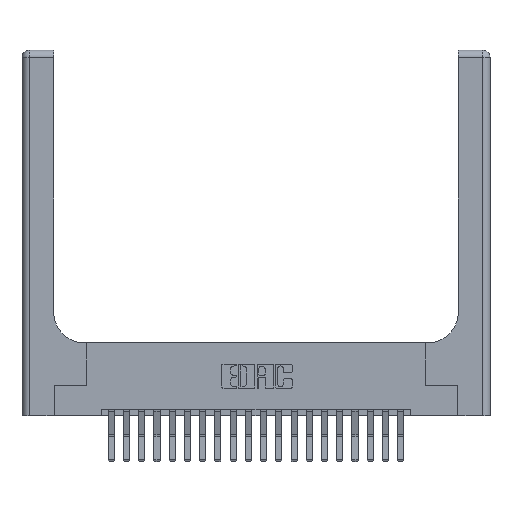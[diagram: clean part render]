
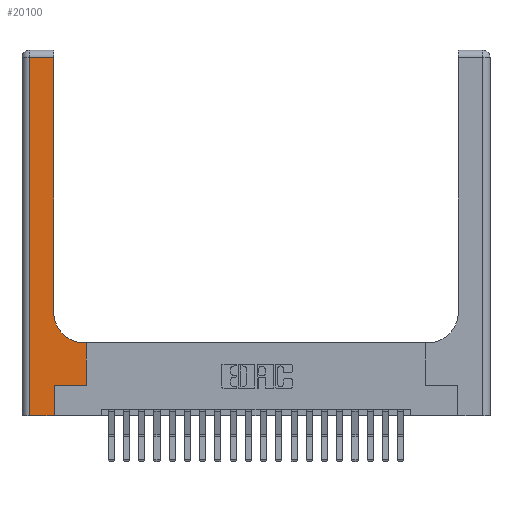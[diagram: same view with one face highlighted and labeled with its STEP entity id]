
A CAD part, top view. The second image highlights one B-rep face of the part: STEP entity #20100.
In plain terms, the highlighted planar face has unit normal (0, 0, 1).
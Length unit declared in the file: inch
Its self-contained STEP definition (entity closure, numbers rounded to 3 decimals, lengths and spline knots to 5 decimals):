
#234 = VECTOR ( 'NONE', #13671, 39.37008 ) ;
#561 = CARTESIAN_POINT ( 'NONE',  ( 0.26, 0.6, 0.37 ) ) ;
#590 = CIRCLE ( 'NONE', #10752, 0.25 ) ;
#679 = VECTOR ( 'NONE', #9015, 39.37008 ) ;
#888 = LINE ( 'NONE', #561, #679 ) ;
#981 = VECTOR ( 'NONE', #6049, 39.37008 ) ;
#1722 = CARTESIAN_POINT ( 'NONE',  ( 0.265, 0., 0.37 ) ) ;
#1819 = VERTEX_POINT ( 'NONE', #3884 ) ;
#2094 = FACE_OUTER_BOUND ( 'NONE', #9244, .T. ) ;
#2648 = CARTESIAN_POINT ( 'NONE',  ( 0., 0., 0.37 ) ) ;
#3008 = DIRECTION ( 'NONE',  ( 1., 0., 0. ) ) ;
#3083 = VERTEX_POINT ( 'NONE', #11999 ) ;
#3443 = VERTEX_POINT ( 'NONE', #10113 ) ;
#3742 = EDGE_CURVE ( 'NONE', #6792, #18751, #6155, .T. ) ;
#3884 = CARTESIAN_POINT ( 'NONE',  ( 0.528, 0.25, 0.37 ) ) ;
#4431 = EDGE_CURVE ( 'NONE', #14919, #6886, #15430, .T. ) ;
#4685 = AXIS2_PLACEMENT_3D ( 'NONE', #8678, #15389, #20233 ) ;
#4989 = EDGE_CURVE ( 'NONE', #3443, #14919, #16165, .T. ) ;
#5001 = ORIENTED_EDGE ( 'NONE', *, *, #4431, .T. ) ;
#5224 = DIRECTION ( 'NONE',  ( 0., 1., 0. ) ) ;
#5262 = ORIENTED_EDGE ( 'NONE', *, *, #3742, .T. ) ;
#5453 = DIRECTION ( 'NONE',  ( 0., 1., 0. ) ) ;
#5541 = EDGE_CURVE ( 'NONE', #6886, #6792, #6564, .T. ) ;
#5683 = EDGE_CURVE ( 'NONE', #1819, #17136, #11819, .T. ) ;
#5905 = ORIENTED_EDGE ( 'NONE', *, *, #11962, .T. ) ;
#6049 = DIRECTION ( 'NONE',  ( 0., 1., 0. ) ) ;
#6155 = LINE ( 'NONE', #2648, #15317 ) ;
#6564 = LINE ( 'NONE', #13371, #17859 ) ;
#6792 = VERTEX_POINT ( 'NONE', #8618 ) ;
#6886 = VERTEX_POINT ( 'NONE', #19608 ) ;
#7027 = EDGE_CURVE ( 'NONE', #3083, #3443, #590, .T. ) ;
#7193 = ORIENTED_EDGE ( 'NONE', *, *, #15438, .T. ) ;
#8172 = CARTESIAN_POINT ( 'NONE',  ( 0.26, 2.94, 0.37 ) ) ;
#8618 = CARTESIAN_POINT ( 'NONE',  ( 0.06, 0., 0.37 ) ) ;
#8678 = CARTESIAN_POINT ( 'NONE',  ( 0., 3., 0.37 ) ) ;
#9015 = DIRECTION ( 'NONE',  ( -1., 0., 0. ) ) ;
#9226 = CARTESIAN_POINT ( 'NONE',  ( 0.26, 3., 0.37 ) ) ;
#9244 = EDGE_LOOP ( 'NONE', ( #19111, #5001, #17368, #5262, #14146, #7193, #20048, #5905, #17726 ) ) ;
#9334 = DIRECTION ( 'NONE',  ( 1., 0., 0. ) ) ;
#10013 = CARTESIAN_POINT ( 'NONE',  ( 0.265, 0.25, 0.37 ) ) ;
#10113 = CARTESIAN_POINT ( 'NONE',  ( 0.26, 0.85, 0.37 ) ) ;
#10190 = VECTOR ( 'NONE', #5224, 39.37008 ) ;
#10411 = CARTESIAN_POINT ( 'NONE',  ( 0.265, 0.25, 0.37 ) ) ;
#10509 = LINE ( 'NONE', #10411, #15478 ) ;
#10752 = AXIS2_PLACEMENT_3D ( 'NONE', #13218, #13107, #3008 ) ;
#11695 = VERTEX_POINT ( 'NONE', #10013 ) ;
#11819 = LINE ( 'NONE', #15132, #21029 ) ;
#11962 = EDGE_CURVE ( 'NONE', #17136, #3083, #888, .T. ) ;
#11999 = CARTESIAN_POINT ( 'NONE',  ( 0.51, 0.6, 0.37 ) ) ;
#13107 = DIRECTION ( 'NONE',  ( 0., 0., -1. ) ) ;
#13218 = CARTESIAN_POINT ( 'NONE',  ( 0.51, 0.85, 0.37 ) ) ;
#13265 = DIRECTION ( 'NONE',  ( 0., -1., 0. ) ) ;
#13371 = CARTESIAN_POINT ( 'NONE',  ( 0.06, 3., 0.37 ) ) ;
#13671 = DIRECTION ( 'NONE',  ( -1., 0., 0. ) ) ;
#14146 = ORIENTED_EDGE ( 'NONE', *, *, #15577, .T. ) ;
#14919 = VERTEX_POINT ( 'NONE', #8172 ) ;
#15132 = CARTESIAN_POINT ( 'NONE',  ( 0.528, 0.25, 0.37 ) ) ;
#15317 = VECTOR ( 'NONE', #9334, 39.37008 ) ;
#15389 = DIRECTION ( 'NONE',  ( 0., 0., -1. ) ) ;
#15430 = LINE ( 'NONE', #17202, #234 ) ;
#15438 = EDGE_CURVE ( 'NONE', #11695, #1819, #10509, .T. ) ;
#15478 = VECTOR ( 'NONE', #18988, 39.37008 ) ;
#15577 = EDGE_CURVE ( 'NONE', #18751, #11695, #16671, .T. ) ;
#16165 = LINE ( 'NONE', #9226, #981 ) ;
#16671 = LINE ( 'NONE', #1722, #10190 ) ;
#16826 = PLANE ( 'NONE',  #4685 ) ;
#17117 = CARTESIAN_POINT ( 'NONE',  ( 0.528, 0.6, 0.37 ) ) ;
#17136 = VERTEX_POINT ( 'NONE', #17117 ) ;
#17202 = CARTESIAN_POINT ( 'NONE',  ( 0., 2.94, 0.37 ) ) ;
#17368 = ORIENTED_EDGE ( 'NONE', *, *, #5541, .T. ) ;
#17726 = ORIENTED_EDGE ( 'NONE', *, *, #7027, .T. ) ;
#17859 = VECTOR ( 'NONE', #13265, 39.37008 ) ;
#18446 = CARTESIAN_POINT ( 'NONE',  ( 0.265, 0., 0.37 ) ) ;
#18751 = VERTEX_POINT ( 'NONE', #18446 ) ;
#18988 = DIRECTION ( 'NONE',  ( 1., 0., 0. ) ) ;
#19111 = ORIENTED_EDGE ( 'NONE', *, *, #4989, .T. ) ;
#19608 = CARTESIAN_POINT ( 'NONE',  ( 0.06, 2.94, 0.37 ) ) ;
#20048 = ORIENTED_EDGE ( 'NONE', *, *, #5683, .T. ) ;
#20100 = ADVANCED_FACE ( 'NONE', ( #2094 ), #16826, .F. ) ;
#20233 = DIRECTION ( 'NONE',  ( -1., 0., 0. ) ) ;
#21029 = VECTOR ( 'NONE', #5453, 39.37008 ) ;
